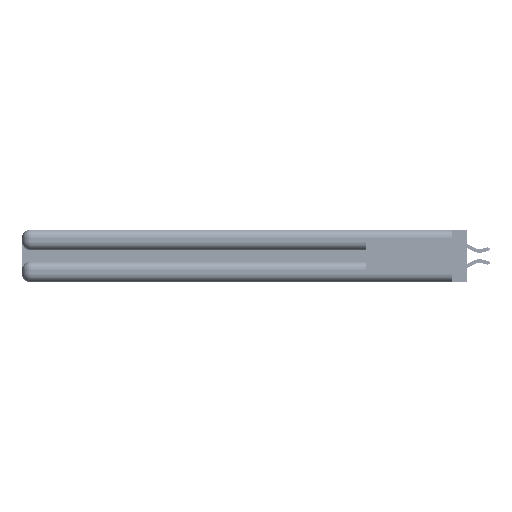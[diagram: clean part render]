
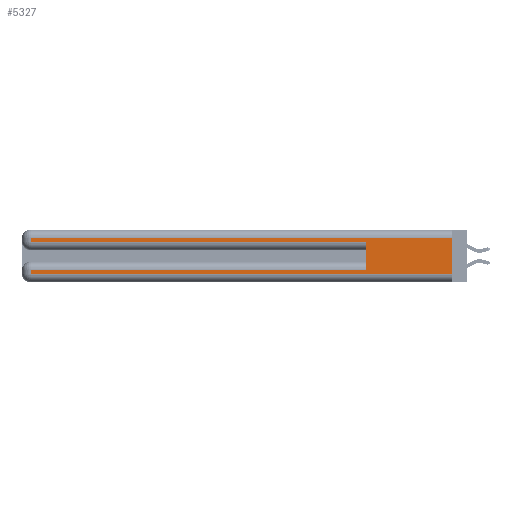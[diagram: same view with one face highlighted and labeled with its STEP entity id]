
A CAD part, left-side view. The second image highlights one B-rep face of the part: STEP entity #5327.
In plain terms, the highlighted planar face has unit normal (-1, 0, 0).
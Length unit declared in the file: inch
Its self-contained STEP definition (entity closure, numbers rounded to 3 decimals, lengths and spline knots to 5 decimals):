
#1871 = CARTESIAN_POINT ( 'NONE',  ( 0., 0., 0.37 ) ) ;
#1940 = LINE ( 'NONE', #21177, #45602 ) ;
#2232 = ORIENTED_EDGE ( 'NONE', *, *, #22324, .T. ) ;
#3413 = CARTESIAN_POINT ( 'NONE',  ( 0., 0., 0.31 ) ) ;
#4094 = CARTESIAN_POINT ( 'NONE',  ( 0., 0., 0.285 ) ) ;
#4267 = LINE ( 'NONE', #7599, #5577 ) ;
#4640 = CARTESIAN_POINT ( 'NONE',  ( 0., 2.94, 0.285 ) ) ;
#5327 = ADVANCED_FACE ( 'NONE', ( #42574 ), #18916, .F. ) ;
#5577 = VECTOR ( 'NONE', #32937, 39.37008 ) ;
#5584 = DIRECTION ( 'NONE',  ( 0., 0., -1. ) ) ;
#6408 = CARTESIAN_POINT ( 'NONE',  ( 0., 0.6, 0.285 ) ) ;
#7153 = VERTEX_POINT ( 'NONE', #10047 ) ;
#7359 = LINE ( 'NONE', #27772, #31187 ) ;
#7495 = LINE ( 'NONE', #4094, #49858 ) ;
#7599 = CARTESIAN_POINT ( 'NONE',  ( 0., 2.94, 0.37 ) ) ;
#10047 = CARTESIAN_POINT ( 'NONE',  ( 0., 2.94, 0.06 ) ) ;
#10745 = DIRECTION ( 'NONE',  ( 0., 1., 0. ) ) ;
#11621 = VERTEX_POINT ( 'NONE', #49960 ) ;
#11629 = VERTEX_POINT ( 'NONE', #12035 ) ;
#12035 = CARTESIAN_POINT ( 'NONE',  ( 0., 2.94, 0.085 ) ) ;
#12821 = DIRECTION ( 'NONE',  ( 0., 0., -1. ) ) ;
#15843 = ORIENTED_EDGE ( 'NONE', *, *, #16309, .T. ) ;
#16309 = EDGE_CURVE ( 'NONE', #49937, #44079, #7495, .T. ) ;
#16617 = LINE ( 'NONE', #16798, #27851 ) ;
#16798 = CARTESIAN_POINT ( 'NONE',  ( 0., 0.6, 0.145 ) ) ;
#18916 = PLANE ( 'NONE',  #39620 ) ;
#19740 = ORIENTED_EDGE ( 'NONE', *, *, #47831, .T. ) ;
#20427 = LINE ( 'NONE', #54129, #41534 ) ;
#20993 = VERTEX_POINT ( 'NONE', #3413 ) ;
#21177 = CARTESIAN_POINT ( 'NONE',  ( 0., 0., 0.37 ) ) ;
#22324 = EDGE_CURVE ( 'NONE', #7153, #11621, #20427, .T. ) ;
#23185 = DIRECTION ( 'NONE',  ( 1., 0., 0. ) ) ;
#24559 = DIRECTION ( 'NONE',  ( 0., -1., 0. ) ) ;
#25370 = VERTEX_POINT ( 'NONE', #52036 ) ;
#25514 = ORIENTED_EDGE ( 'NONE', *, *, #28693, .T. ) ;
#26383 = EDGE_LOOP ( 'NONE', ( #26916, #36228, #43503, #15843, #49005, #25514, #19740, #2232 ) ) ;
#26916 = ORIENTED_EDGE ( 'NONE', *, *, #49290, .F. ) ;
#27772 = CARTESIAN_POINT ( 'NONE',  ( 0., 0., 0.31 ) ) ;
#27851 = VECTOR ( 'NONE', #33614, 39.37008 ) ;
#28693 = EDGE_CURVE ( 'NONE', #25370, #11629, #51762, .T. ) ;
#29302 = VECTOR ( 'NONE', #10745, 39.37008 ) ;
#29446 = EDGE_CURVE ( 'NONE', #20993, #32001, #7359, .T. ) ;
#31187 = VECTOR ( 'NONE', #48863, 39.37008 ) ;
#31440 = VECTOR ( 'NONE', #5584, 39.37008 ) ;
#31815 = CARTESIAN_POINT ( 'NONE',  ( 0., 0., 0.085 ) ) ;
#32001 = VERTEX_POINT ( 'NONE', #44054 ) ;
#32937 = DIRECTION ( 'NONE',  ( 0., 0., -1. ) ) ;
#33614 = DIRECTION ( 'NONE',  ( 0., 0., 1. ) ) ;
#34125 = LINE ( 'NONE', #47788, #31440 ) ;
#36228 = ORIENTED_EDGE ( 'NONE', *, *, #29446, .T. ) ;
#37948 = DIRECTION ( 'NONE',  ( 0., -1., 0. ) ) ;
#39620 = AXIS2_PLACEMENT_3D ( 'NONE', #1871, #23185, #52727 ) ;
#41534 = VECTOR ( 'NONE', #24559, 39.37008 ) ;
#42574 = FACE_OUTER_BOUND ( 'NONE', #26383, .T. ) ;
#43503 = ORIENTED_EDGE ( 'NONE', *, *, #47504, .T. ) ;
#44054 = CARTESIAN_POINT ( 'NONE',  ( 0., 2.94, 0.31 ) ) ;
#44079 = VERTEX_POINT ( 'NONE', #6408 ) ;
#45602 = VECTOR ( 'NONE', #12821, 39.37008 ) ;
#47504 = EDGE_CURVE ( 'NONE', #32001, #49937, #34125, .T. ) ;
#47788 = CARTESIAN_POINT ( 'NONE',  ( 0., 2.94, 0.37 ) ) ;
#47831 = EDGE_CURVE ( 'NONE', #11629, #7153, #4267, .T. ) ;
#48548 = EDGE_CURVE ( 'NONE', #25370, #44079, #16617, .T. ) ;
#48863 = DIRECTION ( 'NONE',  ( 0., 1., 0. ) ) ;
#49005 = ORIENTED_EDGE ( 'NONE', *, *, #48548, .F. ) ;
#49290 = EDGE_CURVE ( 'NONE', #20993, #11621, #1940, .T. ) ;
#49858 = VECTOR ( 'NONE', #37948, 39.37008 ) ;
#49937 = VERTEX_POINT ( 'NONE', #4640 ) ;
#49960 = CARTESIAN_POINT ( 'NONE',  ( 0., 0., 0.06 ) ) ;
#51762 = LINE ( 'NONE', #31815, #29302 ) ;
#52036 = CARTESIAN_POINT ( 'NONE',  ( 0., 0.6, 0.085 ) ) ;
#52727 = DIRECTION ( 'NONE',  ( 0., 0., -1. ) ) ;
#54129 = CARTESIAN_POINT ( 'NONE',  ( 0., 0., 0.06 ) ) ;
